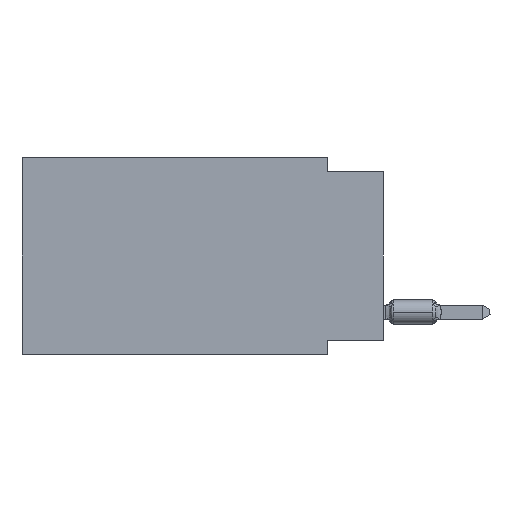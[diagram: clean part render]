
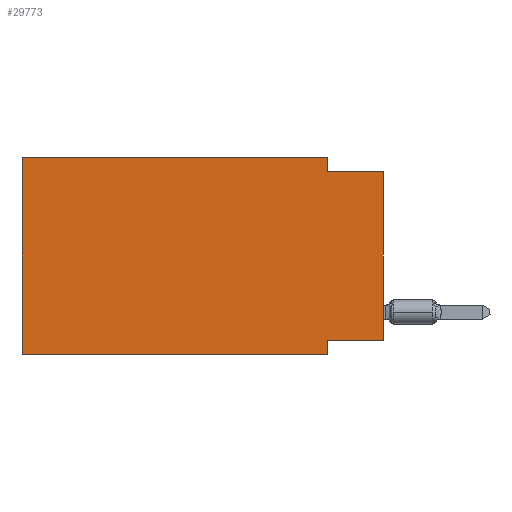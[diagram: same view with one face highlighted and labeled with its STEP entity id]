
A CAD part, left-side view. The second image highlights one B-rep face of the part: STEP entity #29773.
In plain terms, the highlighted planar face has unit normal (-1, 0, 0).
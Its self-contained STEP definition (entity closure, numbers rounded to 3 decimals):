
#4058 = VECTOR ( 'NONE', #13186, 1000. ) ;
#4864 = DIRECTION ( 'NONE',  ( 0., 1., 0. ) ) ;
#5463 = CARTESIAN_POINT ( 'NONE',  ( 0., 16.383, 0. ) ) ;
#6080 = VECTOR ( 'NONE', #96841, 1000. ) ;
#7781 = VERTEX_POINT ( 'NONE', #54095 ) ;
#10323 = VECTOR ( 'NONE', #42685, 1000. ) ;
#11918 = VECTOR ( 'NONE', #114367, 1000. ) ;
#13186 = DIRECTION ( 'NONE',  ( 0., 0., 1. ) ) ;
#21456 = CARTESIAN_POINT ( 'NONE',  ( 0., 2.54, 0. ) ) ;
#22620 = ORIENTED_EDGE ( 'NONE', *, *, #63211, .F. ) ;
#22707 = CARTESIAN_POINT ( 'NONE',  ( 0., 0., 0. ) ) ;
#23524 = VERTEX_POINT ( 'NONE', #21456 ) ;
#24875 = ORIENTED_EDGE ( 'NONE', *, *, #42182, .F. ) ;
#25337 = CARTESIAN_POINT ( 'NONE',  ( 0., 0., -0.635 ) ) ;
#26688 = PLANE ( 'NONE',  #66256 ) ;
#27559 = EDGE_CURVE ( 'NONE', #51034, #33377, #33422, .T. ) ;
#28415 = VERTEX_POINT ( 'NONE', #31505 ) ;
#29773 = ADVANCED_FACE ( 'NONE', ( #44530 ), #26688, .F. ) ;
#30265 = LINE ( 'NONE', #77275, #57440 ) ;
#30560 = LINE ( 'NONE', #31147, #99695 ) ;
#31147 = CARTESIAN_POINT ( 'NONE',  ( 0., 2.54, 0. ) ) ;
#31431 = DIRECTION ( 'NONE',  ( 0., 0., -1. ) ) ;
#31505 = CARTESIAN_POINT ( 'NONE',  ( 0., 16.383, 0. ) ) ;
#31685 = CARTESIAN_POINT ( 'NONE',  ( 0., 0., -8.255 ) ) ;
#33377 = VERTEX_POINT ( 'NONE', #67452 ) ;
#33422 = LINE ( 'NONE', #31685, #94510 ) ;
#41760 = DIRECTION ( 'NONE',  ( 0., -1., 0. ) ) ;
#42104 = CARTESIAN_POINT ( 'NONE',  ( 0., 16.383, -8.89 ) ) ;
#42182 = EDGE_CURVE ( 'NONE', #33377, #69675, #30265, .T. ) ;
#42685 = DIRECTION ( 'NONE',  ( 0., -1., 0. ) ) ;
#44530 = FACE_OUTER_BOUND ( 'NONE', #107940, .T. ) ;
#45536 = CARTESIAN_POINT ( 'NONE',  ( 0., 2.54, -0.635 ) ) ;
#51034 = VERTEX_POINT ( 'NONE', #117013 ) ;
#51617 = LINE ( 'NONE', #42104, #10323 ) ;
#54095 = CARTESIAN_POINT ( 'NONE',  ( 0., 0., -0.635 ) ) ;
#55483 = ORIENTED_EDGE ( 'NONE', *, *, #96423, .T. ) ;
#57440 = VECTOR ( 'NONE', #31431, 1000. ) ;
#63211 = EDGE_CURVE ( 'NONE', #79405, #28415, #86952, .T. ) ;
#66256 = AXIS2_PLACEMENT_3D ( 'NONE', #97567, #79683, #71332 ) ;
#67452 = CARTESIAN_POINT ( 'NONE',  ( 0., 2.54, -8.255 ) ) ;
#67956 = LINE ( 'NONE', #22707, #4058 ) ;
#69675 = VERTEX_POINT ( 'NONE', #88789 ) ;
#70978 = EDGE_CURVE ( 'NONE', #23524, #110184, #30560, .T. ) ;
#71332 = DIRECTION ( 'NONE',  ( 0., 0., -1. ) ) ;
#71759 = CARTESIAN_POINT ( 'NONE',  ( 0., 16.383, -8.89 ) ) ;
#74403 = ORIENTED_EDGE ( 'NONE', *, *, #111140, .F. ) ;
#77275 = CARTESIAN_POINT ( 'NONE',  ( 0., 2.54, -8.89 ) ) ;
#79405 = VERTEX_POINT ( 'NONE', #71759 ) ;
#79683 = DIRECTION ( 'NONE',  ( 1., 0., 0. ) ) ;
#82532 = EDGE_CURVE ( 'NONE', #28415, #23524, #87046, .T. ) ;
#85382 = EDGE_CURVE ( 'NONE', #79405, #69675, #51617, .T. ) ;
#86359 = CARTESIAN_POINT ( 'NONE',  ( 0., 16.383, 0. ) ) ;
#86952 = LINE ( 'NONE', #86359, #11918 ) ;
#87046 = LINE ( 'NONE', #5463, #88009 ) ;
#88009 = VECTOR ( 'NONE', #41760, 1000. ) ;
#88789 = CARTESIAN_POINT ( 'NONE',  ( 0., 2.54, -8.89 ) ) ;
#89705 = ORIENTED_EDGE ( 'NONE', *, *, #70978, .F. ) ;
#94510 = VECTOR ( 'NONE', #4864, 1000. ) ;
#96423 = EDGE_CURVE ( 'NONE', #51034, #7781, #67956, .T. ) ;
#96841 = DIRECTION ( 'NONE',  ( 0., -1., 0. ) ) ;
#97376 = ORIENTED_EDGE ( 'NONE', *, *, #85382, .T. ) ;
#97567 = CARTESIAN_POINT ( 'NONE',  ( 0., 16.383, 0. ) ) ;
#99695 = VECTOR ( 'NONE', #102653, 1000. ) ;
#102653 = DIRECTION ( 'NONE',  ( 0., 0., -1. ) ) ;
#107940 = EDGE_LOOP ( 'NONE', ( #55483, #74403, #89705, #114088, #22620, #97376, #24875, #114418 ) ) ;
#108139 = LINE ( 'NONE', #25337, #6080 ) ;
#110184 = VERTEX_POINT ( 'NONE', #45536 ) ;
#111140 = EDGE_CURVE ( 'NONE', #110184, #7781, #108139, .T. ) ;
#114088 = ORIENTED_EDGE ( 'NONE', *, *, #82532, .F. ) ;
#114367 = DIRECTION ( 'NONE',  ( 0., 0., 1. ) ) ;
#114418 = ORIENTED_EDGE ( 'NONE', *, *, #27559, .F. ) ;
#117013 = CARTESIAN_POINT ( 'NONE',  ( 0., 0., -8.255 ) ) ;
